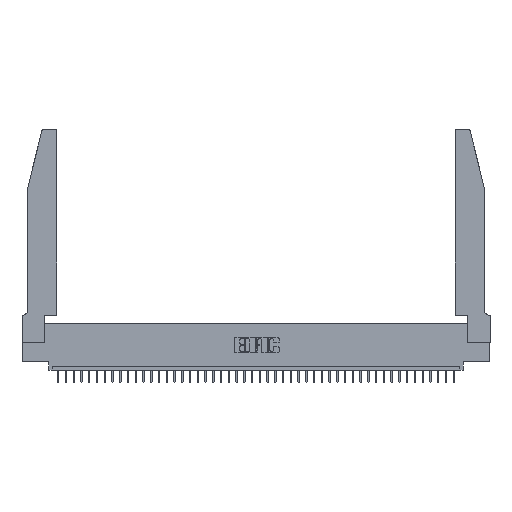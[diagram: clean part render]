
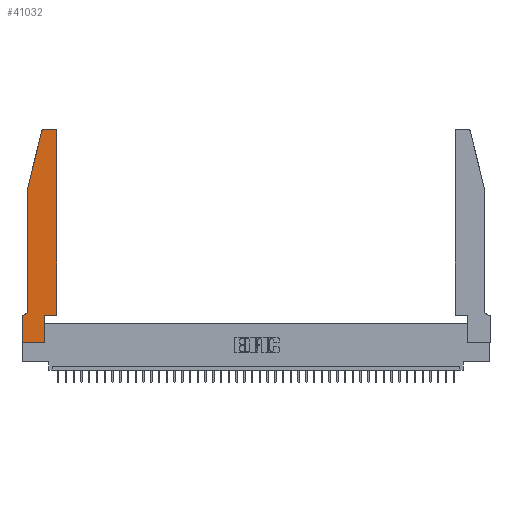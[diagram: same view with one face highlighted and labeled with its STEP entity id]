
A CAD part, top view. The second image highlights one B-rep face of the part: STEP entity #41032.
In plain terms, the highlighted planar face has unit normal (0, 0, 1).
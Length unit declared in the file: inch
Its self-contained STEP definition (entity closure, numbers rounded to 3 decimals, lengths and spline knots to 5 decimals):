
#1271 = EDGE_CURVE ( 'NONE', #41755, #2206, #6898, .T. ) ;
#2206 = VERTEX_POINT ( 'NONE', #30317 ) ;
#2325 = CARTESIAN_POINT ( 'NONE',  ( 0.4205, 2.72, 0.37 ) ) ;
#2426 = VERTEX_POINT ( 'NONE', #36449 ) ;
#2628 = DIRECTION ( 'NONE',  ( 1., 0., 0. ) ) ;
#2891 = DIRECTION ( 'NONE',  ( 0., 0., 1. ) ) ;
#2957 = CARTESIAN_POINT ( 'NONE',  ( 0.284, 2.72, 0.37 ) ) ;
#3209 = DIRECTION ( 'NONE',  ( 0., -1., 0. ) ) ;
#3528 = LINE ( 'NONE', #35941, #27242 ) ;
#4303 = EDGE_CURVE ( 'NONE', #13138, #22314, #10780, .T. ) ;
#4392 = CARTESIAN_POINT ( 'NONE',  ( 0.2865, 0.35, 0.37 ) ) ;
#4694 = CARTESIAN_POINT ( 'NONE',  ( 0.0055, 0.35, 0.37 ) ) ;
#6139 = CARTESIAN_POINT ( 'NONE',  ( 0.0755, 0.42, 0.37 ) ) ;
#6170 = DIRECTION ( 'NONE',  ( 1., 0., 0. ) ) ;
#6249 = DIRECTION ( 'NONE',  ( 0., 0., 1. ) ) ;
#6457 = ORIENTED_EDGE ( 'NONE', *, *, #33811, .T. ) ;
#6898 = LINE ( 'NONE', #15749, #42085 ) ;
#6997 = DIRECTION ( 'NONE',  ( 0., -1., 0. ) ) ;
#8763 = EDGE_CURVE ( 'NONE', #2426, #24211, #37688, .T. ) ;
#8885 = CARTESIAN_POINT ( 'NONE',  ( 0.25487, 2.72718, 0.37 ) ) ;
#9954 = CARTESIAN_POINT ( 'NONE',  ( 0., 0.35, 0.37 ) ) ;
#10165 = DIRECTION ( 'NONE',  ( 0., 0., -1. ) ) ;
#10780 = LINE ( 'NONE', #25601, #29426 ) ;
#11097 = EDGE_CURVE ( 'NONE', #32789, #31191, #14785, .T. ) ;
#11130 = EDGE_LOOP ( 'NONE', ( #24248, #18001, #40412, #32085, #6457, #14536, #30884, #34903, #30444, #41356, #23302, #14521 ) ) ;
#11149 = AXIS2_PLACEMENT_3D ( 'NONE', #2957, #6249, #29316 ) ;
#11934 = VECTOR ( 'NONE', #6997, 39.37008 ) ;
#12314 = VERTEX_POINT ( 'NONE', #21908 ) ;
#13138 = VERTEX_POINT ( 'NONE', #24507 ) ;
#13455 = DIRECTION ( 'NONE',  ( -0.239, -0.971, 0. ) ) ;
#14223 = CARTESIAN_POINT ( 'NONE',  ( 0.0755, 2., 0.37 ) ) ;
#14521 = ORIENTED_EDGE ( 'NONE', *, *, #36789, .T. ) ;
#14536 = ORIENTED_EDGE ( 'NONE', *, *, #21960, .T. ) ;
#14785 = LINE ( 'NONE', #25479, #25603 ) ;
#15048 = CARTESIAN_POINT ( 'NONE',  ( 0., 0., 0.37 ) ) ;
#15709 = DIRECTION ( 'NONE',  ( 1., 0., 0. ) ) ;
#15749 = CARTESIAN_POINT ( 'NONE',  ( 0., 0., 0.37 ) ) ;
#16100 = VECTOR ( 'NONE', #36576, 39.37008 ) ;
#16250 = DIRECTION ( 'NONE',  ( -1., 0., 0. ) ) ;
#16972 = CARTESIAN_POINT ( 'NONE',  ( 0.0755, 0.35, 0.37 ) ) ;
#17925 = VERTEX_POINT ( 'NONE', #4694 ) ;
#18001 = ORIENTED_EDGE ( 'NONE', *, *, #18072, .T. ) ;
#18072 = EDGE_CURVE ( 'NONE', #22314, #29559, #38997, .T. ) ;
#18328 = VERTEX_POINT ( 'NONE', #9954 ) ;
#18572 = DIRECTION ( 'NONE',  ( -1., 0., 0. ) ) ;
#19660 = CARTESIAN_POINT ( 'NONE',  ( 0.0755, 2., 0.37 ) ) ;
#20179 = AXIS2_PLACEMENT_3D ( 'NONE', #32853, #10165, #16250 ) ;
#20723 = EDGE_CURVE ( 'NONE', #29559, #2426, #37818, .T. ) ;
#21021 = DIRECTION ( 'NONE',  ( 0., 0., 1. ) ) ;
#21616 = DIRECTION ( 'NONE',  ( 1., 0., 0. ) ) ;
#21817 = LINE ( 'NONE', #16972, #16100 ) ;
#21908 = CARTESIAN_POINT ( 'NONE',  ( 0.4505, 2.72, 0.37 ) ) ;
#21960 = EDGE_CURVE ( 'NONE', #17925, #18328, #21817, .T. ) ;
#22314 = VERTEX_POINT ( 'NONE', #41965 ) ;
#23302 = ORIENTED_EDGE ( 'NONE', *, *, #36119, .T. ) ;
#24211 = VERTEX_POINT ( 'NONE', #6139 ) ;
#24248 = ORIENTED_EDGE ( 'NONE', *, *, #4303, .T. ) ;
#24507 = CARTESIAN_POINT ( 'NONE',  ( 0.4205, 2.75, 0.37 ) ) ;
#24709 = CIRCLE ( 'NONE', #31953, 0.03 ) ;
#25479 = CARTESIAN_POINT ( 'NONE',  ( 0.4505, 0.35, 0.37 ) ) ;
#25601 = CARTESIAN_POINT ( 'NONE',  ( 0.2605, 2.75, 0.37 ) ) ;
#25603 = VECTOR ( 'NONE', #6170, 39.37008 ) ;
#27242 = VECTOR ( 'NONE', #3209, 39.37008 ) ;
#27557 = EDGE_CURVE ( 'NONE', #18328, #41755, #3528, .T. ) ;
#27570 = CARTESIAN_POINT ( 'NONE',  ( 0.4505, 0.35, 0.37 ) ) ;
#29316 = DIRECTION ( 'NONE',  ( 1., 0., 0. ) ) ;
#29426 = VECTOR ( 'NONE', #18572, 39.37008 ) ;
#29559 = VERTEX_POINT ( 'NONE', #8885 ) ;
#30041 = VECTOR ( 'NONE', #32858, 39.37008 ) ;
#30086 = VECTOR ( 'NONE', #13455, 39.37008 ) ;
#30317 = CARTESIAN_POINT ( 'NONE',  ( 0.2865, 0., 0.37 ) ) ;
#30444 = ORIENTED_EDGE ( 'NONE', *, *, #30697, .T. ) ;
#30697 = EDGE_CURVE ( 'NONE', #2206, #32789, #42030, .T. ) ;
#30884 = ORIENTED_EDGE ( 'NONE', *, *, #27557, .T. ) ;
#31191 = VERTEX_POINT ( 'NONE', #27570 ) ;
#31953 = AXIS2_PLACEMENT_3D ( 'NONE', #2325, #2891, #15709 ) ;
#32085 = ORIENTED_EDGE ( 'NONE', *, *, #8763, .T. ) ;
#32789 = VERTEX_POINT ( 'NONE', #4392 ) ;
#32853 = CARTESIAN_POINT ( 'NONE',  ( 0.0055, 0.42, 0.37 ) ) ;
#32858 = DIRECTION ( 'NONE',  ( 0., 1., 0. ) ) ;
#33487 = VECTOR ( 'NONE', #38550, 39.37008 ) ;
#33811 = EDGE_CURVE ( 'NONE', #24211, #17925, #35265, .T. ) ;
#34539 = AXIS2_PLACEMENT_3D ( 'NONE', #37864, #21021, #21616 ) ;
#34584 = PLANE ( 'NONE',  #34539 ) ;
#34903 = ORIENTED_EDGE ( 'NONE', *, *, #1271, .T. ) ;
#35265 = CIRCLE ( 'NONE', #20179, 0.07 ) ;
#35559 = LINE ( 'NONE', #42069, #33487 ) ;
#35941 = CARTESIAN_POINT ( 'NONE',  ( 0., 0., 0.37 ) ) ;
#36027 = CARTESIAN_POINT ( 'NONE',  ( 0.2865, 0.35, 0.37 ) ) ;
#36119 = EDGE_CURVE ( 'NONE', #31191, #12314, #35559, .T. ) ;
#36449 = CARTESIAN_POINT ( 'NONE',  ( 0.0755, 2., 0.37 ) ) ;
#36576 = DIRECTION ( 'NONE',  ( -1., 0., 0. ) ) ;
#36789 = EDGE_CURVE ( 'NONE', #12314, #13138, #24709, .T. ) ;
#37688 = LINE ( 'NONE', #14223, #11934 ) ;
#37818 = LINE ( 'NONE', #19660, #30086 ) ;
#37864 = CARTESIAN_POINT ( 'NONE',  ( 0., 0.35, 0.37 ) ) ;
#38550 = DIRECTION ( 'NONE',  ( 0., 1., 0. ) ) ;
#38997 = CIRCLE ( 'NONE', #11149, 0.03 ) ;
#40412 = ORIENTED_EDGE ( 'NONE', *, *, #20723, .T. ) ;
#41032 = ADVANCED_FACE ( 'NONE', ( #41408 ), #34584, .T. ) ;
#41356 = ORIENTED_EDGE ( 'NONE', *, *, #11097, .T. ) ;
#41408 = FACE_OUTER_BOUND ( 'NONE', #11130, .T. ) ;
#41755 = VERTEX_POINT ( 'NONE', #15048 ) ;
#41965 = CARTESIAN_POINT ( 'NONE',  ( 0.284, 2.75, 0.37 ) ) ;
#42030 = LINE ( 'NONE', #36027, #30041 ) ;
#42069 = CARTESIAN_POINT ( 'NONE',  ( 0.4505, 0.35, 0.37 ) ) ;
#42085 = VECTOR ( 'NONE', #2628, 39.37008 ) ;
